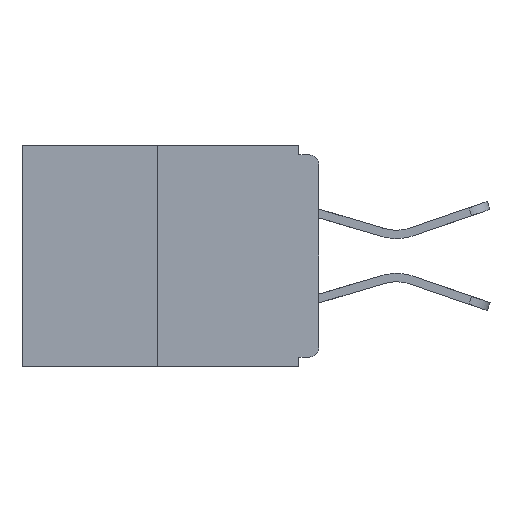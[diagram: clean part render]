
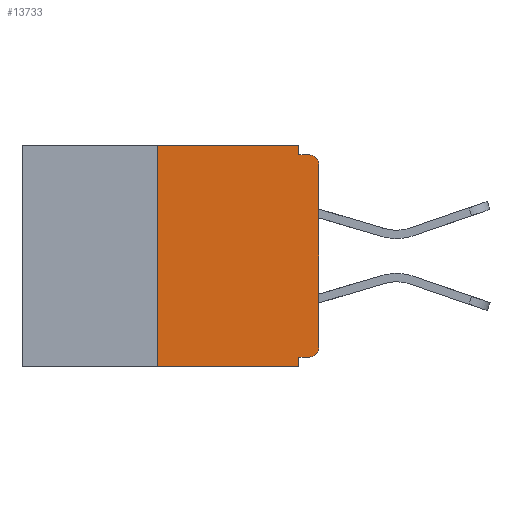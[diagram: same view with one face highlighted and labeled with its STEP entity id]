
A CAD part, left-side view. The second image highlights one B-rep face of the part: STEP entity #13733.
In plain terms, the highlighted planar face has unit normal (-1, 0, 0).
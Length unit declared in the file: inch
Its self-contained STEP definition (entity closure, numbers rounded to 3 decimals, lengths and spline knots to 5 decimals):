
#136 = CARTESIAN_POINT ( 'NONE',  ( 0., 0., 0. ) ) ;
#563 = PLANE ( 'NONE',  #14510 ) ;
#626 = DIRECTION ( 'NONE',  ( 0., 0., -1. ) ) ;
#766 = EDGE_CURVE ( 'NONE', #11578, #13974, #1446, .T. ) ;
#1025 = CARTESIAN_POINT ( 'NONE',  ( 0., 0.25, 0. ) ) ;
#1250 = LINE ( 'NONE', #136, #5908 ) ;
#1381 = CARTESIAN_POINT ( 'NONE',  ( 0., 0.031, -0.015 ) ) ;
#1446 = LINE ( 'NONE', #10897, #15273 ) ;
#1631 = DIRECTION ( 'NONE',  ( 0., -1., 0. ) ) ;
#1767 = VECTOR ( 'NONE', #16088, 39.37008 ) ;
#1985 = DIRECTION ( 'NONE',  ( -1., 0., 0. ) ) ;
#2198 = ORIENTED_EDGE ( 'NONE', *, *, #16539, .F. ) ;
#2630 = CARTESIAN_POINT ( 'NONE',  ( 0., 0.015, -0.015 ) ) ;
#2675 = DIRECTION ( 'NONE',  ( 0., 1., 0. ) ) ;
#2772 = CARTESIAN_POINT ( 'NONE',  ( 0., 0.015, -0.313 ) ) ;
#3034 = CARTESIAN_POINT ( 'NONE',  ( 0., 0., -0.03 ) ) ;
#3148 = VERTEX_POINT ( 'NONE', #4617 ) ;
#3531 = DIRECTION ( 'NONE',  ( 0., -1., 0. ) ) ;
#3576 = EDGE_CURVE ( 'NONE', #3148, #11578, #14100, .T. ) ;
#4216 = LINE ( 'NONE', #8693, #9993 ) ;
#4353 = VERTEX_POINT ( 'NONE', #17469 ) ;
#4364 = DIRECTION ( 'NONE',  ( 0., 0., 1. ) ) ;
#4393 = VERTEX_POINT ( 'NONE', #3034 ) ;
#4617 = CARTESIAN_POINT ( 'NONE',  ( 0., 0.031, 0. ) ) ;
#4861 = CARTESIAN_POINT ( 'NONE',  ( 0., 0.46, 0. ) ) ;
#5368 = VECTOR ( 'NONE', #17628, 39.37008 ) ;
#5408 = ORIENTED_EDGE ( 'NONE', *, *, #766, .F. ) ;
#5470 = CIRCLE ( 'NONE', #5791, 0.015 ) ;
#5791 = AXIS2_PLACEMENT_3D ( 'NONE', #12271, #1985, #17987 ) ;
#5882 = ORIENTED_EDGE ( 'NONE', *, *, #10665, .T. ) ;
#5908 = VECTOR ( 'NONE', #4364, 39.37008 ) ;
#6453 = EDGE_CURVE ( 'NONE', #17867, #13236, #17899, .T. ) ;
#6533 = EDGE_CURVE ( 'NONE', #4353, #6802, #13241, .T. ) ;
#6802 = VERTEX_POINT ( 'NONE', #12022 ) ;
#7110 = CARTESIAN_POINT ( 'NONE',  ( 0., 0.031, 0. ) ) ;
#7315 = LINE ( 'NONE', #8474, #11848 ) ;
#7344 = CARTESIAN_POINT ( 'NONE',  ( 0., 0.25, -0.343 ) ) ;
#7532 = CARTESIAN_POINT ( 'NONE',  ( 0., 0.015, -0.328 ) ) ;
#7795 = EDGE_CURVE ( 'NONE', #13037, #10930, #13641, .T. ) ;
#7800 = ORIENTED_EDGE ( 'NONE', *, *, #6533, .F. ) ;
#7828 = VECTOR ( 'NONE', #16127, 39.37008 ) ;
#7879 = EDGE_CURVE ( 'NONE', #17867, #4353, #7315, .T. ) ;
#8474 = CARTESIAN_POINT ( 'NONE',  ( 0., 0., -0.328 ) ) ;
#8509 = ORIENTED_EDGE ( 'NONE', *, *, #7795, .F. ) ;
#8693 = CARTESIAN_POINT ( 'NONE',  ( 0., 0.46, 0. ) ) ;
#9131 = DIRECTION ( 'NONE',  ( 1., 0., 0. ) ) ;
#9993 = VECTOR ( 'NONE', #1631, 39.37008 ) ;
#10665 = EDGE_CURVE ( 'NONE', #13236, #4393, #1250, .T. ) ;
#10770 = ORIENTED_EDGE ( 'NONE', *, *, #6453, .T. ) ;
#10773 = EDGE_CURVE ( 'NONE', #4393, #13974, #5470, .T. ) ;
#10897 = CARTESIAN_POINT ( 'NONE',  ( 0., 0., -0.015 ) ) ;
#10930 = VERTEX_POINT ( 'NONE', #1025 ) ;
#11255 = VECTOR ( 'NONE', #3531, 39.37008 ) ;
#11578 = VERTEX_POINT ( 'NONE', #1381 ) ;
#11817 = ORIENTED_EDGE ( 'NONE', *, *, #7879, .F. ) ;
#11848 = VECTOR ( 'NONE', #2675, 39.37008 ) ;
#12022 = CARTESIAN_POINT ( 'NONE',  ( 0., 0.031, -0.343 ) ) ;
#12163 = FACE_OUTER_BOUND ( 'NONE', #12382, .T. ) ;
#12271 = CARTESIAN_POINT ( 'NONE',  ( 0., 0.015, -0.03 ) ) ;
#12357 = DIRECTION ( 'NONE',  ( 0., -1., 0. ) ) ;
#12382 = EDGE_LOOP ( 'NONE', ( #2198, #8509, #17557, #7800, #11817, #10770, #5882, #15388, #5408, #16193 ) ) ;
#12810 = DIRECTION ( 'NONE',  ( -1., 0., 0. ) ) ;
#13037 = VERTEX_POINT ( 'NONE', #7344 ) ;
#13236 = VERTEX_POINT ( 'NONE', #13773 ) ;
#13241 = LINE ( 'NONE', #17572, #7828 ) ;
#13558 = CARTESIAN_POINT ( 'NONE',  ( 0., 0.25, 0. ) ) ;
#13602 = EDGE_CURVE ( 'NONE', #13037, #6802, #15044, .T. ) ;
#13641 = LINE ( 'NONE', #13558, #1767 ) ;
#13733 = ADVANCED_FACE ( 'NONE', ( #12163 ), #563, .F. ) ;
#13773 = CARTESIAN_POINT ( 'NONE',  ( 0., 0., -0.313 ) ) ;
#13974 = VERTEX_POINT ( 'NONE', #2630 ) ;
#14100 = LINE ( 'NONE', #7110, #5368 ) ;
#14236 = DIRECTION ( 'NONE',  ( 0., 0., -1. ) ) ;
#14510 = AXIS2_PLACEMENT_3D ( 'NONE', #4861, #9131, #626 ) ;
#15037 = CARTESIAN_POINT ( 'NONE',  ( 0., 0.46, -0.343 ) ) ;
#15044 = LINE ( 'NONE', #15037, #11255 ) ;
#15213 = AXIS2_PLACEMENT_3D ( 'NONE', #2772, #12810, #14236 ) ;
#15273 = VECTOR ( 'NONE', #12357, 39.37008 ) ;
#15388 = ORIENTED_EDGE ( 'NONE', *, *, #10773, .T. ) ;
#16088 = DIRECTION ( 'NONE',  ( 0., 0., 1. ) ) ;
#16127 = DIRECTION ( 'NONE',  ( 0., 0., -1. ) ) ;
#16193 = ORIENTED_EDGE ( 'NONE', *, *, #3576, .F. ) ;
#16539 = EDGE_CURVE ( 'NONE', #10930, #3148, #4216, .T. ) ;
#17469 = CARTESIAN_POINT ( 'NONE',  ( 0., 0.031, -0.328 ) ) ;
#17557 = ORIENTED_EDGE ( 'NONE', *, *, #13602, .T. ) ;
#17572 = CARTESIAN_POINT ( 'NONE',  ( 0., 0.031, -0.343 ) ) ;
#17628 = DIRECTION ( 'NONE',  ( 0., 0., -1. ) ) ;
#17867 = VERTEX_POINT ( 'NONE', #7532 ) ;
#17899 = CIRCLE ( 'NONE', #15213, 0.015 ) ;
#17987 = DIRECTION ( 'NONE',  ( 0., 0., -1. ) ) ;
